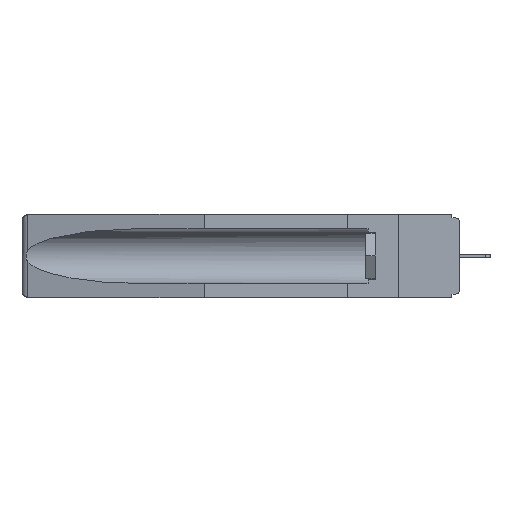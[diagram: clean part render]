
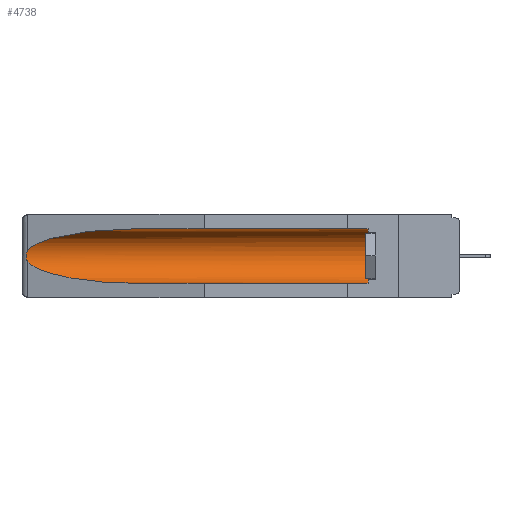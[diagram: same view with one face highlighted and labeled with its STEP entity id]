
A CAD part, left-side view. The second image highlights one B-rep face of the part: STEP entity #4738.
In plain terms, the highlighted cylindrical face has radius 2.857 mm (diameter 5.715 mm), a partial arc.
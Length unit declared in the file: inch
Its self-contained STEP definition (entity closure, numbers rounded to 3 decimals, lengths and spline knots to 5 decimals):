
#977 = AXIS2_PLACEMENT_3D ( 'NONE', #6120, #2111, #14039 ) ;
#1305 = FACE_OUTER_BOUND ( 'NONE', #3451, .T. ) ;
#1804 = CARTESIAN_POINT ( 'NONE',  ( 0.155, 0.126, -0.059 ) ) ;
#1855 = VERTEX_POINT ( 'NONE', #8847 ) ;
#2111 = DIRECTION ( 'NONE',  ( 0., 1., 0. ) ) ;
#2346 = CARTESIAN_POINT ( 'NONE',  ( 0.2675, 1.53308, -0.16763 ) ) ;
#2690 = VECTOR ( 'NONE', #18186, 39.37008 ) ;
#2926 = EDGE_CURVE ( 'NONE', #12298, #1855, #12275, .T. ) ;
#2957 = EDGE_CURVE ( 'NONE', #3829, #3174, #14317, .T. ) ;
#3041 = CARTESIAN_POINT ( 'NONE',  ( 0.26537, 1.52718, -0.14972 ) ) ;
#3174 = VERTEX_POINT ( 'NONE', #1804 ) ;
#3451 = EDGE_LOOP ( 'NONE', ( #7087, #6553, #5496, #3762, #8391, #7604 ) ) ;
#3508 = CARTESIAN_POINT ( 'NONE',  ( 0.155, 0.126, -0.284 ) ) ;
#3603 = CARTESIAN_POINT ( 'NONE',  ( 0.155, -0.30754, -0.059 ) ) ;
#3762 = ORIENTED_EDGE ( 'NONE', *, *, #5066, .F. ) ;
#3829 = VERTEX_POINT ( 'NONE', #3508 ) ;
#3843 = CARTESIAN_POINT ( 'NONE',  ( 0.26654, 1.53092, -0.15636 ) ) ;
#4403 = CARTESIAN_POINT ( 'NONE',  ( 0.155, 1.07973, -0.059 ) ) ;
#4738 = ADVANCED_FACE ( 'NONE', ( #1305 ), #18815, .F. ) ;
#5066 = EDGE_CURVE ( 'NONE', #3829, #5702, #6637, .T. ) ;
#5091 = DIRECTION ( 'NONE',  ( 0., 1., 0. ) ) ;
#5496 = ORIENTED_EDGE ( 'NONE', *, *, #7949, .T. ) ;
#5702 = VERTEX_POINT ( 'NONE', #12485 ) ;
#6120 = CARTESIAN_POINT ( 'NONE',  ( 0.155, -0.30754, -0.1715 ) ) ;
#6235 = CARTESIAN_POINT ( 'NONE',  ( 0.155, -0.30754, -0.284 ) ) ;
#6553 = ORIENTED_EDGE ( 'NONE', *, *, #2926, .T. ) ;
#6637 = LINE ( 'NONE', #6235, #2690 ) ;
#6743 = CARTESIAN_POINT ( 'NONE',  ( 0.2673, 1.5327, -0.16383 ) ) ;
#6873 = CARTESIAN_POINT ( 'NONE',  ( 0.26655, 1.53094, -0.18657 ) ) ;
#7087 = ORIENTED_EDGE ( 'NONE', *, *, #13169, .T. ) ;
#7604 = ORIENTED_EDGE ( 'NONE', *, *, #12443, .T. ) ;
#7949 = EDGE_CURVE ( 'NONE', #1855, #5702, #16839, .T. ) ;
#7960 = CARTESIAN_POINT ( 'NONE',  ( 0.21114, 1.30732, -0.284 ) ) ;
#8319 = CARTESIAN_POINT ( 'NONE',  ( 0.2675, 1.53308, -0.17534 ) ) ;
#8391 = ORIENTED_EDGE ( 'NONE', *, *, #2957, .T. ) ;
#8847 = CARTESIAN_POINT ( 'NONE',  ( 0.26537, 1.52718, -0.19328 ) ) ;
#10409 = CARTESIAN_POINT ( 'NONE',  ( 0.26537, 1.52718, -0.19328 ) ) ;
#10669 = LINE ( 'NONE', #3603, #12036 ) ;
#10954 = CARTESIAN_POINT ( 'NONE',  ( 0.25451, 1.48313, -0.24835 ) ) ;
#11489 = DIRECTION ( 'NONE',  ( 0., -1., 0. ) ) ;
#11933 = CARTESIAN_POINT ( 'NONE',  ( 0.155, 1.07973, -0.284 ) ) ;
#12036 = VECTOR ( 'NONE', #5091, 39.37008 ) ;
#12171 = CARTESIAN_POINT ( 'NONE',  ( 0.26537, 1.52718, -0.14972 ) ) ;
#12275 = B_SPLINE_CURVE_WITH_KNOTS ( 'NONE', 3,
 ( #14083, #15529, #3843, #6743, #2346, #8319, #15670, #6873, #17140, #12779 ),
 .UNSPECIFIED., .F., .F.,
 ( 4, 2, 2, 2, 4 ),
 ( 0., 0.00029, 0.00058, 0.00087, 0.00117 ),
 .UNSPECIFIED. ) ;
#12298 = VERTEX_POINT ( 'NONE', #12171 ) ;
#12443 = EDGE_CURVE ( 'NONE', #3174, #16213, #10669, .T. ) ;
#12485 = CARTESIAN_POINT ( 'NONE',  ( 0.155, 1.07973, -0.284 ) ) ;
#12779 = CARTESIAN_POINT ( 'NONE',  ( 0.26537, 1.52718, -0.19328 ) ) ;
#13141 = CARTESIAN_POINT ( 'NONE',  ( 0.25451, 1.48313, -0.09465 ) ) ;
#13169 = EDGE_CURVE ( 'NONE', #16213, #12298, #15896, .T. ) ;
#14039 = DIRECTION ( 'NONE',  ( 0., 0., 1. ) ) ;
#14083 = CARTESIAN_POINT ( 'NONE',  ( 0.26537, 1.52718, -0.14972 ) ) ;
#14317 = CIRCLE ( 'NONE', #18787, 0.1125 ) ;
#14679 = CARTESIAN_POINT ( 'NONE',  ( 0.21114, 1.30732, -0.059 ) ) ;
#15529 = CARTESIAN_POINT ( 'NONE',  ( 0.26597, 1.52961, -0.15275 ) ) ;
#15670 = CARTESIAN_POINT ( 'NONE',  ( 0.2673, 1.53269, -0.17917 ) ) ;
#15779 = CARTESIAN_POINT ( 'NONE',  ( 0.155, 0.126, -0.1715 ) ) ;
#15896 =( BOUNDED_CURVE ( )  B_SPLINE_CURVE ( 3, ( #4403, #14679, #13141, #3041 ),
 .UNSPECIFIED., .F., .T. ) 
 B_SPLINE_CURVE_WITH_KNOTS ( ( 4, 4 ),
 ( 4.71239, 6.08839 ),
 .UNSPECIFIED. ) 
 CURVE ( )  GEOMETRIC_REPRESENTATION_ITEM ( )  RATIONAL_B_SPLINE_CURVE ( ( 1., 0.848, 0.848, 1. ) ) 
 REPRESENTATION_ITEM ( '' )  );
#16213 = VERTEX_POINT ( 'NONE', #17830 ) ;
#16839 =( BOUNDED_CURVE ( )  B_SPLINE_CURVE ( 3, ( #10409, #10954, #7960, #11933 ),
 .UNSPECIFIED., .F., .T. ) 
 B_SPLINE_CURVE_WITH_KNOTS ( ( 4, 4 ),
 ( 0.1948, 1.5708 ),
 .UNSPECIFIED. ) 
 CURVE ( )  GEOMETRIC_REPRESENTATION_ITEM ( )  RATIONAL_B_SPLINE_CURVE ( ( 1., 0.848, 0.848, 1. ) ) 
 REPRESENTATION_ITEM ( '' )  );
#17140 = CARTESIAN_POINT ( 'NONE',  ( 0.26597, 1.5296, -0.19026 ) ) ;
#17275 = DIRECTION ( 'NONE',  ( 0., 0., 1. ) ) ;
#17830 = CARTESIAN_POINT ( 'NONE',  ( 0.155, 1.07973, -0.059 ) ) ;
#18186 = DIRECTION ( 'NONE',  ( 0., 1., 0. ) ) ;
#18787 = AXIS2_PLACEMENT_3D ( 'NONE', #15779, #11489, #17275 ) ;
#18815 = CYLINDRICAL_SURFACE ( 'NONE', #977, 0.1125 ) ;
